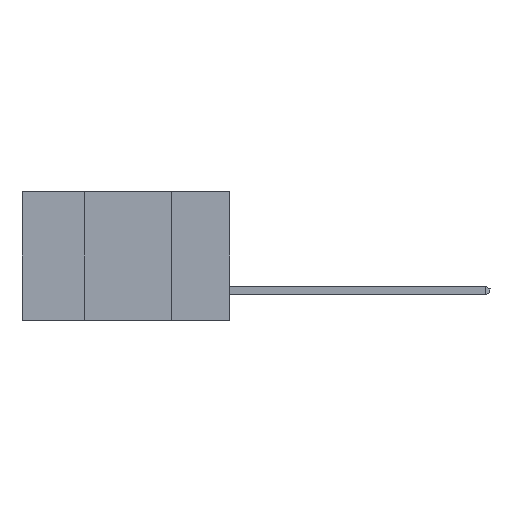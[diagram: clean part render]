
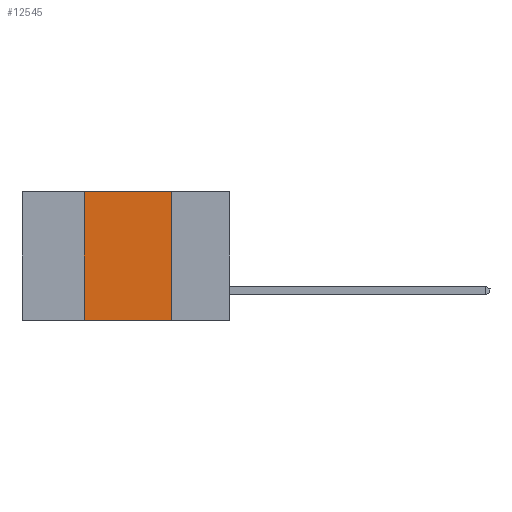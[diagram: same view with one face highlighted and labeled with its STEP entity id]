
A CAD part, left-side view. The second image highlights one B-rep face of the part: STEP entity #12545.
In plain terms, the highlighted planar face has unit normal (-1, 0, 0).
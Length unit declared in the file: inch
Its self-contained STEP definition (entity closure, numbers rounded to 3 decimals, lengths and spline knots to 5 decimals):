
#185 = CARTESIAN_POINT ( 'NONE',  ( 0., 0.17, -0.37 ) ) ;
#359 = DIRECTION ( 'NONE',  ( 0., -1., 0. ) ) ;
#3515 = EDGE_CURVE ( 'NONE', #12252, #15745, #14026, .T. ) ;
#3652 = CARTESIAN_POINT ( 'NONE',  ( 0., 0.6, 0. ) ) ;
#6058 = CARTESIAN_POINT ( 'NONE',  ( 0., 0.17, 0. ) ) ;
#6070 = DIRECTION ( 'NONE',  ( 0., -1., 0. ) ) ;
#7057 = AXIS2_PLACEMENT_3D ( 'NONE', #3652, #21254, #7943 ) ;
#7651 = ORIENTED_EDGE ( 'NONE', *, *, #18335, .T. ) ;
#7943 = DIRECTION ( 'NONE',  ( 0., 0., -1. ) ) ;
#9903 = LINE ( 'NONE', #185, #15997 ) ;
#10216 = VERTEX_POINT ( 'NONE', #6058 ) ;
#12022 = CARTESIAN_POINT ( 'NONE',  ( 0., 0.6, -0.37 ) ) ;
#12252 = VERTEX_POINT ( 'NONE', #24262 ) ;
#12261 = CARTESIAN_POINT ( 'NONE',  ( 0., 0.17, -0.37 ) ) ;
#12545 = ADVANCED_FACE ( 'NONE', ( #19328 ), #25278, .F. ) ;
#14026 = LINE ( 'NONE', #21906, #15008 ) ;
#14151 = DIRECTION ( 'NONE',  ( 0., 0., 1. ) ) ;
#14317 = CARTESIAN_POINT ( 'NONE',  ( 0., 0.42, 0. ) ) ;
#15008 = VECTOR ( 'NONE', #14151, 39.37008 ) ;
#15041 = ORIENTED_EDGE ( 'NONE', *, *, #21913, .F. ) ;
#15745 = VERTEX_POINT ( 'NONE', #14317 ) ;
#15997 = VECTOR ( 'NONE', #19604, 39.37008 ) ;
#16295 = VECTOR ( 'NONE', #359, 39.37008 ) ;
#17850 = CARTESIAN_POINT ( 'NONE',  ( 0., 0.6, 0. ) ) ;
#18335 = EDGE_CURVE ( 'NONE', #12252, #24070, #21849, .T. ) ;
#19328 = FACE_OUTER_BOUND ( 'NONE', #20257, .T. ) ;
#19604 = DIRECTION ( 'NONE',  ( 0., 0., -1. ) ) ;
#20006 = EDGE_CURVE ( 'NONE', #15745, #10216, #21592, .T. ) ;
#20257 = EDGE_LOOP ( 'NONE', ( #15041, #23978, #23079, #7651 ) ) ;
#21254 = DIRECTION ( 'NONE',  ( 1., 0., 0. ) ) ;
#21592 = LINE ( 'NONE', #17850, #22969 ) ;
#21849 = LINE ( 'NONE', #12022, #16295 ) ;
#21906 = CARTESIAN_POINT ( 'NONE',  ( 0., 0.42, -0.37 ) ) ;
#21913 = EDGE_CURVE ( 'NONE', #10216, #24070, #9903, .T. ) ;
#22969 = VECTOR ( 'NONE', #6070, 39.37008 ) ;
#23079 = ORIENTED_EDGE ( 'NONE', *, *, #3515, .F. ) ;
#23978 = ORIENTED_EDGE ( 'NONE', *, *, #20006, .F. ) ;
#24070 = VERTEX_POINT ( 'NONE', #12261 ) ;
#24262 = CARTESIAN_POINT ( 'NONE',  ( 0., 0.42, -0.37 ) ) ;
#25278 = PLANE ( 'NONE',  #7057 ) ;
